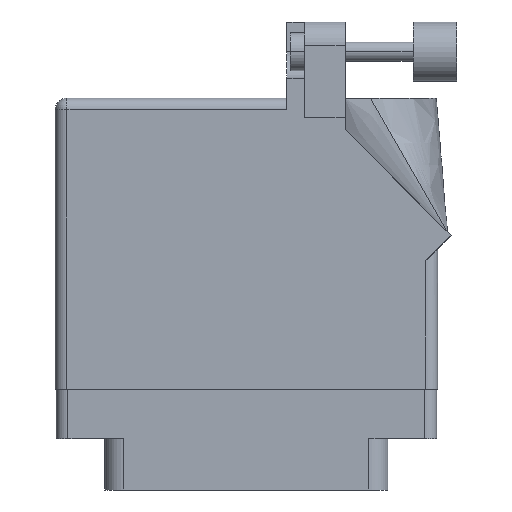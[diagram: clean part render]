
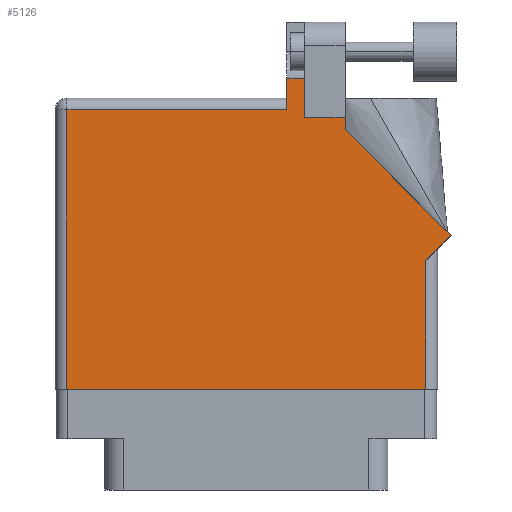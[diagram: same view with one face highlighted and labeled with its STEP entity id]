
A CAD part, front view. The second image highlights one B-rep face of the part: STEP entity #5126.
In plain terms, the highlighted face is planar.
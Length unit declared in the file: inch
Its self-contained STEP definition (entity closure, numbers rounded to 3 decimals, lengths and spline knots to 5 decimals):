
#20 = ORIENTED_EDGE ( 'NONE', *, *, #984, .T. ) ;
#83 = CARTESIAN_POINT ( 'NONE',  ( 1.524, 1.36442, 0. ) ) ;
#890 = CARTESIAN_POINT ( 'NONE',  ( 1.311, 1.43, 0. ) ) ;
#984 = EDGE_CURVE ( 'NONE', #10359, #18041, #32665, .T. ) ;
#1692 = VERTEX_POINT ( 'NONE', #23462 ) ;
#1950 = EDGE_CURVE ( 'NONE', #6478, #25490, #6582, .T. ) ;
#2279 = DIRECTION ( 'NONE',  ( -1., 0., 0. ) ) ;
#2736 = LINE ( 'NONE', #7761, #34255 ) ;
#2776 = EDGE_CURVE ( 'NONE', #32563, #24305, #4424, .T. ) ;
#2841 = ORIENTED_EDGE ( 'NONE', *, *, #8472, .T. ) ;
#3094 = EDGE_LOOP ( 'NONE', ( #5913, #28793, #20, #28691, #35273, #25469, #22710, #15057, #16075, #2841, #14921 ) ) ;
#3209 = EDGE_CURVE ( 'NONE', #11305, #10359, #2736, .T. ) ;
#3463 = DIRECTION ( 'NONE',  ( 0., 1., 0. ) ) ;
#3487 = EDGE_CURVE ( 'NONE', #11488, #32563, #13807, .T. ) ;
#4424 = LINE ( 'NONE', #32691, #35102 ) ;
#4501 = LINE ( 'NONE', #890, #33450 ) ;
#4778 = DIRECTION ( 'NONE',  ( 0., -1., 0. ) ) ;
#4858 = CARTESIAN_POINT ( 'NONE',  ( 0.062, 1.468, 0. ) ) ;
#4894 = CARTESIAN_POINT ( 'NONE',  ( 1.217, 1.6315, 0. ) ) ;
#5126 = ADVANCED_FACE ( 'NONE', ( #30277 ), #6999, .F. ) ;
#5128 = DIRECTION ( 'NONE',  ( 0., -1., 0. ) ) ;
#5142 = VECTOR ( 'NONE', #34134, 39.37008 ) ;
#5388 = DIRECTION ( 'NONE',  ( -1., 0., 0. ) ) ;
#5913 = ORIENTED_EDGE ( 'NONE', *, *, #12530, .T. ) ;
#6478 = VERTEX_POINT ( 'NONE', #29389 ) ;
#6582 = LINE ( 'NONE', #33893, #31753 ) ;
#6999 = PLANE ( 'NONE',  #23676 ) ;
#7647 = VECTOR ( 'NONE', #31634, 39.37008 ) ;
#7761 = CARTESIAN_POINT ( 'NONE',  ( 1.64177, 1.6315, 0. ) ) ;
#8472 = EDGE_CURVE ( 'NONE', #9194, #6478, #10872, .T. ) ;
#8742 = VECTOR ( 'NONE', #16155, 39.37008 ) ;
#9010 = CARTESIAN_POINT ( 'NONE',  ( 1.948, 0.675, 0. ) ) ;
#9194 = VERTEX_POINT ( 'NONE', #83 ) ;
#9285 = DIRECTION ( 'NONE',  ( -1., 0., 0. ) ) ;
#9493 = CARTESIAN_POINT ( 'NONE',  ( 0.062, 0., 0. ) ) ;
#9517 = VECTOR ( 'NONE', #4778, 39.37008 ) ;
#10359 = VERTEX_POINT ( 'NONE', #4894 ) ;
#10698 = CARTESIAN_POINT ( 'NONE',  ( 1.524, 1.36442, 0. ) ) ;
#10872 = LINE ( 'NONE', #10698, #8742 ) ;
#11043 = LINE ( 'NONE', #17959, #13159 ) ;
#11297 = EDGE_CURVE ( 'NONE', #1692, #9194, #19638, .T. ) ;
#11305 = VERTEX_POINT ( 'NONE', #20231 ) ;
#11488 = VERTEX_POINT ( 'NONE', #4858 ) ;
#12530 = EDGE_CURVE ( 'NONE', #25490, #11305, #4501, .T. ) ;
#13159 = VECTOR ( 'NONE', #20836, 39.37008 ) ;
#13647 = DIRECTION ( 'NONE',  ( 1., 0., 0. ) ) ;
#13807 = LINE ( 'NONE', #31576, #9517 ) ;
#14921 = ORIENTED_EDGE ( 'NONE', *, *, #1950, .T. ) ;
#15057 = ORIENTED_EDGE ( 'NONE', *, *, #20706, .T. ) ;
#15586 = DIRECTION ( 'NONE',  ( 0., 0., -1. ) ) ;
#16075 = ORIENTED_EDGE ( 'NONE', *, *, #11297, .T. ) ;
#16155 = DIRECTION ( 'NONE',  ( 0., 1., 0. ) ) ;
#17959 = CARTESIAN_POINT ( 'NONE',  ( 2.01, 0.737, 0. ) ) ;
#18041 = VERTEX_POINT ( 'NONE', #19164 ) ;
#19164 = CARTESIAN_POINT ( 'NONE',  ( 1.217, 1.468, 0. ) ) ;
#19638 = LINE ( 'NONE', #25846, #5142 ) ;
#20231 = CARTESIAN_POINT ( 'NONE',  ( 1.311, 1.6315, 0. ) ) ;
#20706 = EDGE_CURVE ( 'NONE', #28073, #1692, #11043, .T. ) ;
#20836 = DIRECTION ( 'NONE',  ( 0.707, 0.707, 0. ) ) ;
#22545 = LINE ( 'NONE', #34359, #7647 ) ;
#22710 = ORIENTED_EDGE ( 'NONE', *, *, #32638, .T. ) ;
#23305 = VECTOR ( 'NONE', #5128, 39.37008 ) ;
#23462 = CARTESIAN_POINT ( 'NONE',  ( 2.08071, 0.80771, 0. ) ) ;
#23471 = CARTESIAN_POINT ( 'NONE',  ( 1.217, 1.53, 0. ) ) ;
#23676 = AXIS2_PLACEMENT_3D ( 'NONE', #26563, #15586, #2279 ) ;
#24305 = VERTEX_POINT ( 'NONE', #31656 ) ;
#24921 = VECTOR ( 'NONE', #9285, 39.37008 ) ;
#25469 = ORIENTED_EDGE ( 'NONE', *, *, #2776, .T. ) ;
#25490 = VERTEX_POINT ( 'NONE', #27088 ) ;
#25504 = CARTESIAN_POINT ( 'NONE',  ( 0., 1.468, 0. ) ) ;
#25846 = CARTESIAN_POINT ( 'NONE',  ( 2.08071, 0.80771, 0. ) ) ;
#26563 = CARTESIAN_POINT ( 'NONE',  ( 0., 1.53, 0. ) ) ;
#27038 = LINE ( 'NONE', #25504, #24921 ) ;
#27088 = CARTESIAN_POINT ( 'NONE',  ( 1.311, 1.43, 0. ) ) ;
#28073 = VERTEX_POINT ( 'NONE', #9010 ) ;
#28691 = ORIENTED_EDGE ( 'NONE', *, *, #29305, .T. ) ;
#28793 = ORIENTED_EDGE ( 'NONE', *, *, #3209, .T. ) ;
#29305 = EDGE_CURVE ( 'NONE', #18041, #11488, #27038, .T. ) ;
#29389 = CARTESIAN_POINT ( 'NONE',  ( 1.524, 1.43, 0. ) ) ;
#30277 = FACE_OUTER_BOUND ( 'NONE', #3094, .T. ) ;
#31576 = CARTESIAN_POINT ( 'NONE',  ( 0.062, 0., 0. ) ) ;
#31634 = DIRECTION ( 'NONE',  ( 0., 1., 0. ) ) ;
#31656 = CARTESIAN_POINT ( 'NONE',  ( 1.948, 0., 0. ) ) ;
#31753 = VECTOR ( 'NONE', #34011, 39.37008 ) ;
#32563 = VERTEX_POINT ( 'NONE', #9493 ) ;
#32638 = EDGE_CURVE ( 'NONE', #24305, #28073, #22545, .T. ) ;
#32665 = LINE ( 'NONE', #23471, #23305 ) ;
#32691 = CARTESIAN_POINT ( 'NONE',  ( 0., 0., 0. ) ) ;
#33450 = VECTOR ( 'NONE', #3463, 39.37008 ) ;
#33893 = CARTESIAN_POINT ( 'NONE',  ( 1.524, 1.43, 0. ) ) ;
#34011 = DIRECTION ( 'NONE',  ( -1., 0., 0. ) ) ;
#34134 = DIRECTION ( 'NONE',  ( -0.707, 0.707, 0. ) ) ;
#34255 = VECTOR ( 'NONE', #5388, 39.37008 ) ;
#34359 = CARTESIAN_POINT ( 'NONE',  ( 1.948, 0.737, 0. ) ) ;
#35102 = VECTOR ( 'NONE', #13647, 39.37008 ) ;
#35273 = ORIENTED_EDGE ( 'NONE', *, *, #3487, .T. ) ;
